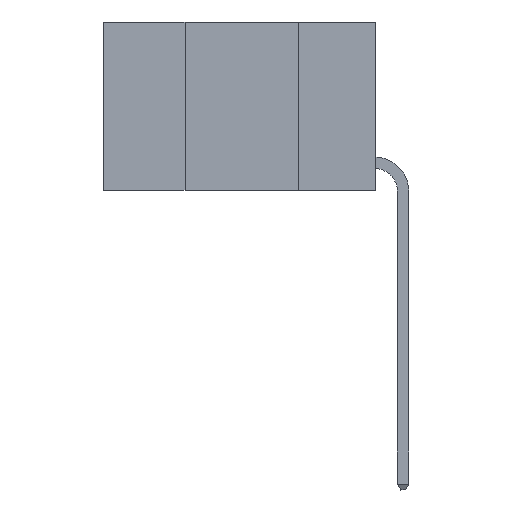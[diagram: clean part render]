
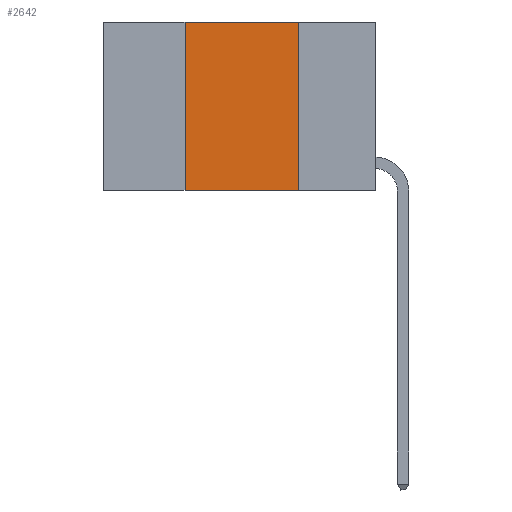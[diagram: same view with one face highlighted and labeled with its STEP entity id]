
A CAD part, left-side view. The second image highlights one B-rep face of the part: STEP entity #2642.
In plain terms, the highlighted planar face has unit normal (-1, 0, 0).
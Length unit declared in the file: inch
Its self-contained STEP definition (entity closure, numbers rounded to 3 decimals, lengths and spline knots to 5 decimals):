
#243 = CARTESIAN_POINT ( 'NONE',  ( 0., 0.42, 0. ) ) ;
#256 = CARTESIAN_POINT ( 'NONE',  ( 0., 0.6, 0. ) ) ;
#854 = EDGE_CURVE ( 'NONE', #5435, #1982, #7628, .T. ) ;
#995 = EDGE_CURVE ( 'NONE', #5435, #3768, #9990, .T. ) ;
#1377 = PLANE ( 'NONE',  #3159 ) ;
#1427 = VERTEX_POINT ( 'NONE', #2788 ) ;
#1982 = VERTEX_POINT ( 'NONE', #7545 ) ;
#2350 = FACE_OUTER_BOUND ( 'NONE', #5697, .T. ) ;
#2460 = VECTOR ( 'NONE', #10096, 39.37008 ) ;
#2466 = DIRECTION ( 'NONE',  ( 0., 0., -1. ) ) ;
#2642 = ADVANCED_FACE ( 'NONE', ( #2350 ), #1377, .F. ) ;
#2653 = VECTOR ( 'NONE', #10309, 39.37008 ) ;
#2788 = CARTESIAN_POINT ( 'NONE',  ( 0., 0.17, 0. ) ) ;
#3159 = AXIS2_PLACEMENT_3D ( 'NONE', #4145, #6813, #3957 ) ;
#3239 = CARTESIAN_POINT ( 'NONE',  ( 0., 0.6, -0.37 ) ) ;
#3768 = VERTEX_POINT ( 'NONE', #6082 ) ;
#3957 = DIRECTION ( 'NONE',  ( 0., 0., -1. ) ) ;
#4006 = DIRECTION ( 'NONE',  ( 0., -1., 0. ) ) ;
#4145 = CARTESIAN_POINT ( 'NONE',  ( 0., 0.6, 0. ) ) ;
#4979 = EDGE_CURVE ( 'NONE', #3768, #1427, #9348, .T. ) ;
#5435 = VERTEX_POINT ( 'NONE', #9998 ) ;
#5437 = VECTOR ( 'NONE', #4006, 39.37008 ) ;
#5680 = ORIENTED_EDGE ( 'NONE', *, *, #995, .F. ) ;
#5697 = EDGE_LOOP ( 'NONE', ( #6312, #8982, #5680, #7451 ) ) ;
#6075 = LINE ( 'NONE', #7795, #11276 ) ;
#6082 = CARTESIAN_POINT ( 'NONE',  ( 0., 0.42, 0. ) ) ;
#6312 = ORIENTED_EDGE ( 'NONE', *, *, #10948, .F. ) ;
#6813 = DIRECTION ( 'NONE',  ( 1., 0., 0. ) ) ;
#7451 = ORIENTED_EDGE ( 'NONE', *, *, #854, .T. ) ;
#7545 = CARTESIAN_POINT ( 'NONE',  ( 0., 0.17, -0.37 ) ) ;
#7628 = LINE ( 'NONE', #3239, #2653 ) ;
#7795 = CARTESIAN_POINT ( 'NONE',  ( 0., 0.17, 0. ) ) ;
#8982 = ORIENTED_EDGE ( 'NONE', *, *, #4979, .F. ) ;
#9348 = LINE ( 'NONE', #256, #5437 ) ;
#9990 = LINE ( 'NONE', #243, #2460 ) ;
#9998 = CARTESIAN_POINT ( 'NONE',  ( 0., 0.42, -0.37 ) ) ;
#10096 = DIRECTION ( 'NONE',  ( 0., 0., 1. ) ) ;
#10309 = DIRECTION ( 'NONE',  ( 0., -1., 0. ) ) ;
#10948 = EDGE_CURVE ( 'NONE', #1427, #1982, #6075, .T. ) ;
#11276 = VECTOR ( 'NONE', #2466, 39.37008 ) ;
